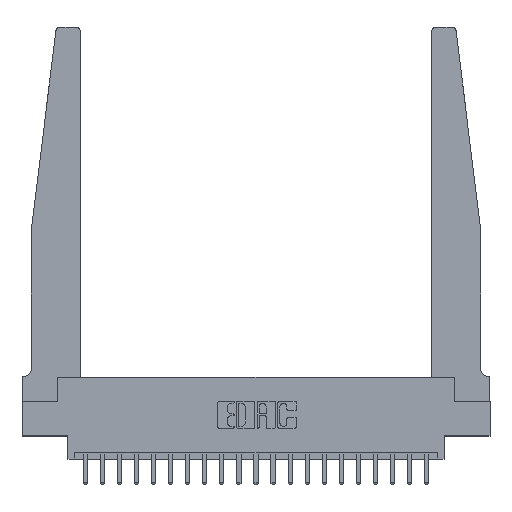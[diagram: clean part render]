
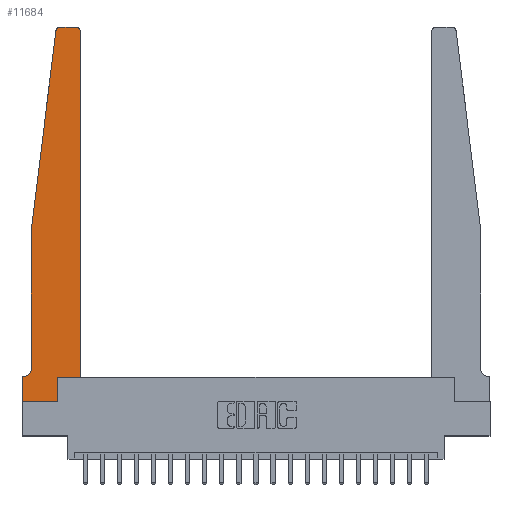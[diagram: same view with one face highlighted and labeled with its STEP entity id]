
A CAD part, top view. The second image highlights one B-rep face of the part: STEP entity #11684.
In plain terms, the highlighted planar face has unit normal (0, 0, 1).
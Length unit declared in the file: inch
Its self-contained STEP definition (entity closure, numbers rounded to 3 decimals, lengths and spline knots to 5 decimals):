
#41 = VERTEX_POINT ( 'NONE', #16395 ) ;
#264 = CARTESIAN_POINT ( 'NONE',  ( 0.2605, 0., 0.37 ) ) ;
#907 = AXIS2_PLACEMENT_3D ( 'NONE', #20505, #12054, #18831 ) ;
#1142 = DIRECTION ( 'NONE',  ( 0., 1., 0. ) ) ;
#1185 = DIRECTION ( 'NONE',  ( 1., 0., 0. ) ) ;
#1373 = VECTOR ( 'NONE', #15373, 39.37008 ) ;
#1663 = VERTEX_POINT ( 'NONE', #8824 ) ;
#1984 = AXIS2_PLACEMENT_3D ( 'NONE', #2395, #8954, #2284 ) ;
#2188 = DIRECTION ( 'NONE',  ( -0.122, -0.992, 0. ) ) ;
#2240 = DIRECTION ( 'NONE',  ( 0., 0., -1. ) ) ;
#2284 = DIRECTION ( 'NONE',  ( 1., 0., 0. ) ) ;
#2350 = ORIENTED_EDGE ( 'NONE', *, *, #5552, .T. ) ;
#2395 = CARTESIAN_POINT ( 'NONE',  ( 0., 0.1875, 0.37 ) ) ;
#2488 = LINE ( 'NONE', #14068, #19398 ) ;
#2634 = CARTESIAN_POINT ( 'NONE',  ( 0.425, 0.18, 0.37 ) ) ;
#3597 = EDGE_CURVE ( 'NONE', #18296, #16739, #5853, .T. ) ;
#3644 = VECTOR ( 'NONE', #20447, 39.37008 ) ;
#3771 = ORIENTED_EDGE ( 'NONE', *, *, #17788, .T. ) ;
#4487 = VERTEX_POINT ( 'NONE', #18794 ) ;
#4672 = AXIS2_PLACEMENT_3D ( 'NONE', #7689, #2240, #11459 ) ;
#4730 = VERTEX_POINT ( 'NONE', #7869 ) ;
#5236 = CARTESIAN_POINT ( 'NONE',  ( 0., 0.1875, 0.37 ) ) ;
#5247 = CARTESIAN_POINT ( 'NONE',  ( 0., 0., 0.37 ) ) ;
#5444 = LINE ( 'NONE', #16773, #3644 ) ;
#5552 = EDGE_CURVE ( 'NONE', #41, #17218, #14176, .T. ) ;
#5678 = VECTOR ( 'NONE', #14828, 39.37008 ) ;
#5738 = DIRECTION ( 'NONE',  ( -1., 0., 0. ) ) ;
#5772 = CARTESIAN_POINT ( 'NONE',  ( 0.27653, 2.75, 0.37 ) ) ;
#5853 = CIRCLE ( 'NONE', #6198, 0.03 ) ;
#5869 = ORIENTED_EDGE ( 'NONE', *, *, #9583, .T. ) ;
#6198 = AXIS2_PLACEMENT_3D ( 'NONE', #7864, #8082, #1185 ) ;
#6279 = CIRCLE ( 'NONE', #907, 0.03 ) ;
#6800 = CARTESIAN_POINT ( 'NONE',  ( 0.425, 2.72, 0.37 ) ) ;
#6893 = EDGE_CURVE ( 'NONE', #16153, #12855, #2488, .T. ) ;
#7071 = EDGE_CURVE ( 'NONE', #9893, #4730, #6279, .T. ) ;
#7081 = DIRECTION ( 'NONE',  ( 1., 0., 0. ) ) ;
#7254 = LINE ( 'NONE', #17259, #20915 ) ;
#7689 = CARTESIAN_POINT ( 'NONE',  ( 0.015, 0.2375, 0.37 ) ) ;
#7817 = EDGE_CURVE ( 'NONE', #8323, #16153, #9231, .T. ) ;
#7864 = CARTESIAN_POINT ( 'NONE',  ( 0.395, 2.72, 0.37 ) ) ;
#7869 = CARTESIAN_POINT ( 'NONE',  ( 0.24675, 2.72367, 0.37 ) ) ;
#8029 = LINE ( 'NONE', #20050, #5678 ) ;
#8082 = DIRECTION ( 'NONE',  ( 0., 0., 1. ) ) ;
#8288 = ORIENTED_EDGE ( 'NONE', *, *, #19683, .T. ) ;
#8323 = VERTEX_POINT ( 'NONE', #13662 ) ;
#8617 = EDGE_CURVE ( 'NONE', #4730, #1663, #14100, .T. ) ;
#8801 = CARTESIAN_POINT ( 'NONE',  ( 0.425, 0.18, 0.37 ) ) ;
#8824 = CARTESIAN_POINT ( 'NONE',  ( 0.065, 1.25, 0.37 ) ) ;
#8933 = CARTESIAN_POINT ( 'NONE',  ( 0.425, 0.18, 0.37 ) ) ;
#8954 = DIRECTION ( 'NONE',  ( 0., 0., 1. ) ) ;
#8976 = VERTEX_POINT ( 'NONE', #264 ) ;
#9231 = CIRCLE ( 'NONE', #4672, 0.05 ) ;
#9278 = EDGE_CURVE ( 'NONE', #12855, #4487, #20478, .T. ) ;
#9379 = FACE_OUTER_BOUND ( 'NONE', #17138, .T. ) ;
#9583 = EDGE_CURVE ( 'NONE', #1663, #8323, #5444, .T. ) ;
#9893 = VERTEX_POINT ( 'NONE', #5772 ) ;
#10125 = LINE ( 'NONE', #8801, #1373 ) ;
#10351 = DIRECTION ( 'NONE',  ( 1., 0., 0. ) ) ;
#11057 = VECTOR ( 'NONE', #18806, 39.37008 ) ;
#11459 = DIRECTION ( 'NONE',  ( -1., 0., 0. ) ) ;
#11600 = VECTOR ( 'NONE', #7081, 39.37008 ) ;
#11684 = ADVANCED_FACE ( 'NONE', ( #9379 ), #19182, .T. ) ;
#12054 = DIRECTION ( 'NONE',  ( 0., 0., 1. ) ) ;
#12519 = CARTESIAN_POINT ( 'NONE',  ( 0.015, 0.1875, 0.37 ) ) ;
#12855 = VERTEX_POINT ( 'NONE', #5236 ) ;
#13434 = EDGE_CURVE ( 'NONE', #16739, #9893, #8029, .T. ) ;
#13588 = CARTESIAN_POINT ( 'NONE',  ( 0.395, 2.75, 0.37 ) ) ;
#13662 = CARTESIAN_POINT ( 'NONE',  ( 0.065, 0.2375, 0.37 ) ) ;
#14068 = CARTESIAN_POINT ( 'NONE',  ( 0.065, 0.1875, 0.37 ) ) ;
#14100 = LINE ( 'NONE', #17424, #15696 ) ;
#14176 = LINE ( 'NONE', #8933, #11600 ) ;
#14828 = DIRECTION ( 'NONE',  ( -1., 0., 0. ) ) ;
#14843 = LINE ( 'NONE', #19720, #19325 ) ;
#15303 = ORIENTED_EDGE ( 'NONE', *, *, #7817, .T. ) ;
#15373 = DIRECTION ( 'NONE',  ( 0., 1., 0. ) ) ;
#15551 = ORIENTED_EDGE ( 'NONE', *, *, #6893, .T. ) ;
#15696 = VECTOR ( 'NONE', #2188, 39.37008 ) ;
#16153 = VERTEX_POINT ( 'NONE', #12519 ) ;
#16395 = CARTESIAN_POINT ( 'NONE',  ( 0.2605, 0.18, 0.37 ) ) ;
#16739 = VERTEX_POINT ( 'NONE', #13588 ) ;
#16773 = CARTESIAN_POINT ( 'NONE',  ( 0.065, 1.25, 0.37 ) ) ;
#17138 = EDGE_LOOP ( 'NONE', ( #20442, #21307, #21055, #5869, #15303, #15551, #19884, #17432, #8288, #2350, #3771, #18325 ) ) ;
#17218 = VERTEX_POINT ( 'NONE', #2634 ) ;
#17259 = CARTESIAN_POINT ( 'NONE',  ( 0., 0., 0.37 ) ) ;
#17424 = CARTESIAN_POINT ( 'NONE',  ( 0.065, 1.25, 0.37 ) ) ;
#17432 = ORIENTED_EDGE ( 'NONE', *, *, #17824, .T. ) ;
#17788 = EDGE_CURVE ( 'NONE', #17218, #18296, #10125, .T. ) ;
#17824 = EDGE_CURVE ( 'NONE', #4487, #8976, #7254, .T. ) ;
#18296 = VERTEX_POINT ( 'NONE', #6800 ) ;
#18325 = ORIENTED_EDGE ( 'NONE', *, *, #3597, .T. ) ;
#18794 = CARTESIAN_POINT ( 'NONE',  ( 0., 0., 0.37 ) ) ;
#18806 = DIRECTION ( 'NONE',  ( 0., -1., 0. ) ) ;
#18831 = DIRECTION ( 'NONE',  ( 1., 0., 0. ) ) ;
#19182 = PLANE ( 'NONE',  #1984 ) ;
#19325 = VECTOR ( 'NONE', #1142, 39.37008 ) ;
#19398 = VECTOR ( 'NONE', #5738, 39.37008 ) ;
#19683 = EDGE_CURVE ( 'NONE', #8976, #41, #14843, .T. ) ;
#19720 = CARTESIAN_POINT ( 'NONE',  ( 0.2605, 0.18, 0.37 ) ) ;
#19884 = ORIENTED_EDGE ( 'NONE', *, *, #9278, .T. ) ;
#20050 = CARTESIAN_POINT ( 'NONE',  ( 0.25, 2.75, 0.37 ) ) ;
#20442 = ORIENTED_EDGE ( 'NONE', *, *, #13434, .T. ) ;
#20447 = DIRECTION ( 'NONE',  ( 0., -1., 0. ) ) ;
#20478 = LINE ( 'NONE', #5247, #11057 ) ;
#20505 = CARTESIAN_POINT ( 'NONE',  ( 0.27653, 2.72, 0.37 ) ) ;
#20915 = VECTOR ( 'NONE', #10351, 39.37008 ) ;
#21055 = ORIENTED_EDGE ( 'NONE', *, *, #8617, .T. ) ;
#21307 = ORIENTED_EDGE ( 'NONE', *, *, #7071, .T. ) ;
